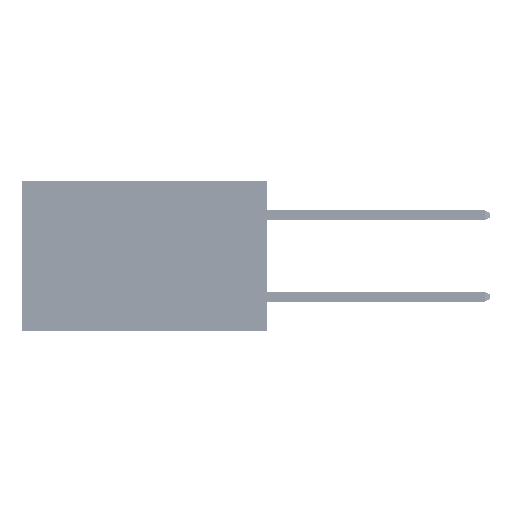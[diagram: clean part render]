
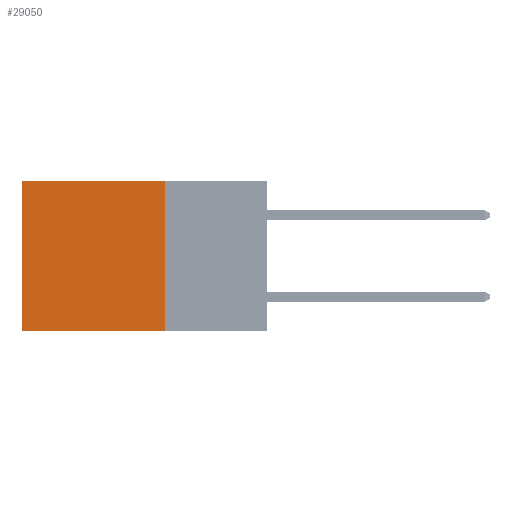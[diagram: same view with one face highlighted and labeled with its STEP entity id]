
A CAD part, left-side view. The second image highlights one B-rep face of the part: STEP entity #29050.
In plain terms, the highlighted planar face has unit normal (-1, 0, 0).
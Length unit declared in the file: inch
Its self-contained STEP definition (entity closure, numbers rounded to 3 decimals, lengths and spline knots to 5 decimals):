
#1286 = LINE ( 'NONE', #45846, #27859 ) ;
#3384 = EDGE_CURVE ( 'NONE', #42496, #36863, #29374, .T. ) ;
#4575 = VECTOR ( 'NONE', #32681, 39.37008 ) ;
#4822 = LINE ( 'NONE', #5933, #13955 ) ;
#5933 = CARTESIAN_POINT ( 'NONE',  ( 0.2875, 0.25, -0.37 ) ) ;
#7075 = VERTEX_POINT ( 'NONE', #38645 ) ;
#9968 = VECTOR ( 'NONE', #21956, 39.37008 ) ;
#12131 = VERTEX_POINT ( 'NONE', #37245 ) ;
#12461 = ORIENTED_EDGE ( 'NONE', *, *, #17947, .T. ) ;
#13748 = CARTESIAN_POINT ( 'NONE',  ( 0.2875, 0.25, 0. ) ) ;
#13860 = ORIENTED_EDGE ( 'NONE', *, *, #28883, .T. ) ;
#13955 = VECTOR ( 'NONE', #14053, 39.37008 ) ;
#14053 = DIRECTION ( 'NONE',  ( 0., 1., 0. ) ) ;
#14936 = EDGE_CURVE ( 'NONE', #36863, #7075, #4822, .T. ) ;
#16345 = DIRECTION ( 'NONE',  ( 0., 1., 0. ) ) ;
#17491 = AXIS2_PLACEMENT_3D ( 'NONE', #13748, #17935, #22084 ) ;
#17935 = DIRECTION ( 'NONE',  ( 1., 0., 0. ) ) ;
#17947 = EDGE_CURVE ( 'NONE', #12131, #7075, #45429, .T. ) ;
#18809 = CARTESIAN_POINT ( 'NONE',  ( 0.2875, 0.25, 0. ) ) ;
#21956 = DIRECTION ( 'NONE',  ( 0., 0., -1. ) ) ;
#22084 = DIRECTION ( 'NONE',  ( 0., 0., -1. ) ) ;
#27859 = VECTOR ( 'NONE', #16345, 39.37008 ) ;
#28883 = EDGE_CURVE ( 'NONE', #42496, #12131, #1286, .T. ) ;
#29050 = ADVANCED_FACE ( 'NONE', ( #49932 ), #38366, .F. ) ;
#29374 = LINE ( 'NONE', #42617, #9968 ) ;
#32681 = DIRECTION ( 'NONE',  ( 0., 0., -1. ) ) ;
#34987 = CARTESIAN_POINT ( 'NONE',  ( 0.2875, 0.25, -0.37 ) ) ;
#36863 = VERTEX_POINT ( 'NONE', #34987 ) ;
#37053 = CARTESIAN_POINT ( 'NONE',  ( 0.2875, 0.6, 0. ) ) ;
#37245 = CARTESIAN_POINT ( 'NONE',  ( 0.2875, 0.6, 0. ) ) ;
#38366 = PLANE ( 'NONE',  #17491 ) ;
#38645 = CARTESIAN_POINT ( 'NONE',  ( 0.2875, 0.6, -0.37 ) ) ;
#38896 = ORIENTED_EDGE ( 'NONE', *, *, #14936, .F. ) ;
#40088 = EDGE_LOOP ( 'NONE', ( #12461, #38896, #51706, #13860 ) ) ;
#42496 = VERTEX_POINT ( 'NONE', #18809 ) ;
#42617 = CARTESIAN_POINT ( 'NONE',  ( 0.2875, 0.25, 0. ) ) ;
#45429 = LINE ( 'NONE', #37053, #4575 ) ;
#45846 = CARTESIAN_POINT ( 'NONE',  ( 0.2875, 0.25, 0. ) ) ;
#49932 = FACE_OUTER_BOUND ( 'NONE', #40088, .T. ) ;
#51706 = ORIENTED_EDGE ( 'NONE', *, *, #3384, .F. ) ;
